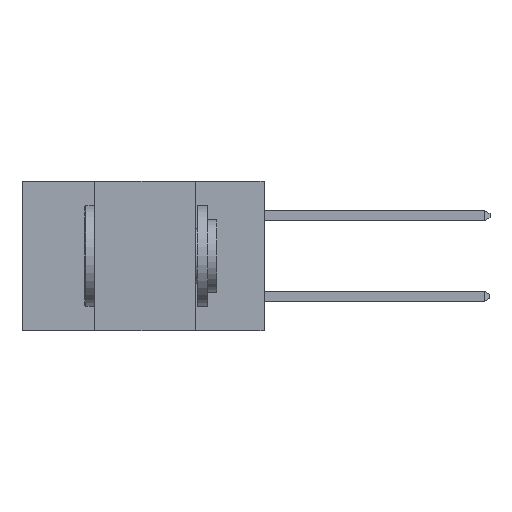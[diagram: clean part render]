
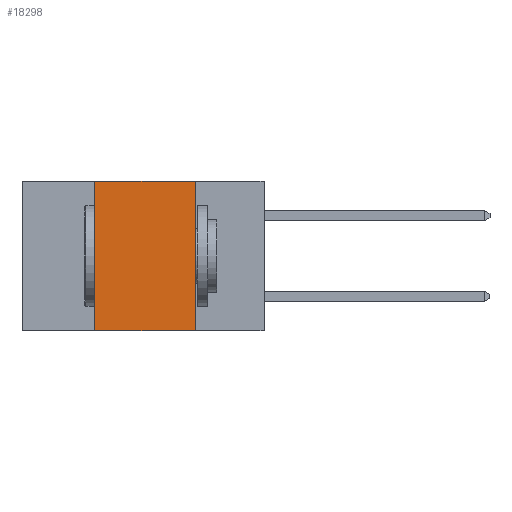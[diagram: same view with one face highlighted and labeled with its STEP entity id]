
A CAD part, left-side view. The second image highlights one B-rep face of the part: STEP entity #18298.
In plain terms, the highlighted planar face has unit normal (-1, 0, 0).
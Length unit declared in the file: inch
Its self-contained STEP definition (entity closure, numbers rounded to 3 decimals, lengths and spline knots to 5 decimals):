
#69 = ORIENTED_EDGE ( 'NONE', *, *, #8942, .F. ) ;
#1164 = CARTESIAN_POINT ( 'NONE',  ( 0., 0.42, 0. ) ) ;
#1315 = LINE ( 'NONE', #10481, #16157 ) ;
#2637 = VERTEX_POINT ( 'NONE', #12325 ) ;
#2841 = ORIENTED_EDGE ( 'NONE', *, *, #12734, .F. ) ;
#3061 = DIRECTION ( 'NONE',  ( 1., 0., 0. ) ) ;
#3911 = VERTEX_POINT ( 'NONE', #10778 ) ;
#4059 = CARTESIAN_POINT ( 'NONE',  ( 0., 0.17, 0. ) ) ;
#4498 = CARTESIAN_POINT ( 'NONE',  ( 0., 0.42, 0. ) ) ;
#5751 = LINE ( 'NONE', #1164, #9246 ) ;
#7223 = ORIENTED_EDGE ( 'NONE', *, *, #16316, .T. ) ;
#7490 = LINE ( 'NONE', #18322, #14920 ) ;
#7730 = CARTESIAN_POINT ( 'NONE',  ( 0., 0.17, 0. ) ) ;
#8629 = DIRECTION ( 'NONE',  ( 0., 0., 1. ) ) ;
#8639 = LINE ( 'NONE', #4059, #12591 ) ;
#8942 = EDGE_CURVE ( 'NONE', #9351, #16387, #7490, .T. ) ;
#9246 = VECTOR ( 'NONE', #8629, 39.37008 ) ;
#9351 = VERTEX_POINT ( 'NONE', #4498 ) ;
#9618 = AXIS2_PLACEMENT_3D ( 'NONE', #14866, #3061, #13451 ) ;
#10481 = CARTESIAN_POINT ( 'NONE',  ( 0., 0.6, -0.37 ) ) ;
#10778 = CARTESIAN_POINT ( 'NONE',  ( 0., 0.42, -0.37 ) ) ;
#10982 = DIRECTION ( 'NONE',  ( 0., -1., 0. ) ) ;
#12022 = DIRECTION ( 'NONE',  ( 0., -1., 0. ) ) ;
#12325 = CARTESIAN_POINT ( 'NONE',  ( 0., 0.17, -0.37 ) ) ;
#12373 = EDGE_LOOP ( 'NONE', ( #2841, #69, #16998, #7223 ) ) ;
#12591 = VECTOR ( 'NONE', #14407, 39.37008 ) ;
#12734 = EDGE_CURVE ( 'NONE', #16387, #2637, #8639, .T. ) ;
#13451 = DIRECTION ( 'NONE',  ( 0., 0., -1. ) ) ;
#14407 = DIRECTION ( 'NONE',  ( 0., 0., -1. ) ) ;
#14477 = FACE_OUTER_BOUND ( 'NONE', #12373, .T. ) ;
#14717 = EDGE_CURVE ( 'NONE', #3911, #9351, #5751, .T. ) ;
#14866 = CARTESIAN_POINT ( 'NONE',  ( 0., 0.6, 0. ) ) ;
#14920 = VECTOR ( 'NONE', #10982, 39.37008 ) ;
#16157 = VECTOR ( 'NONE', #12022, 39.37008 ) ;
#16316 = EDGE_CURVE ( 'NONE', #3911, #2637, #1315, .T. ) ;
#16387 = VERTEX_POINT ( 'NONE', #7730 ) ;
#16998 = ORIENTED_EDGE ( 'NONE', *, *, #14717, .F. ) ;
#17810 = PLANE ( 'NONE',  #9618 ) ;
#18298 = ADVANCED_FACE ( 'NONE', ( #14477 ), #17810, .F. ) ;
#18322 = CARTESIAN_POINT ( 'NONE',  ( 0., 0.6, 0. ) ) ;
